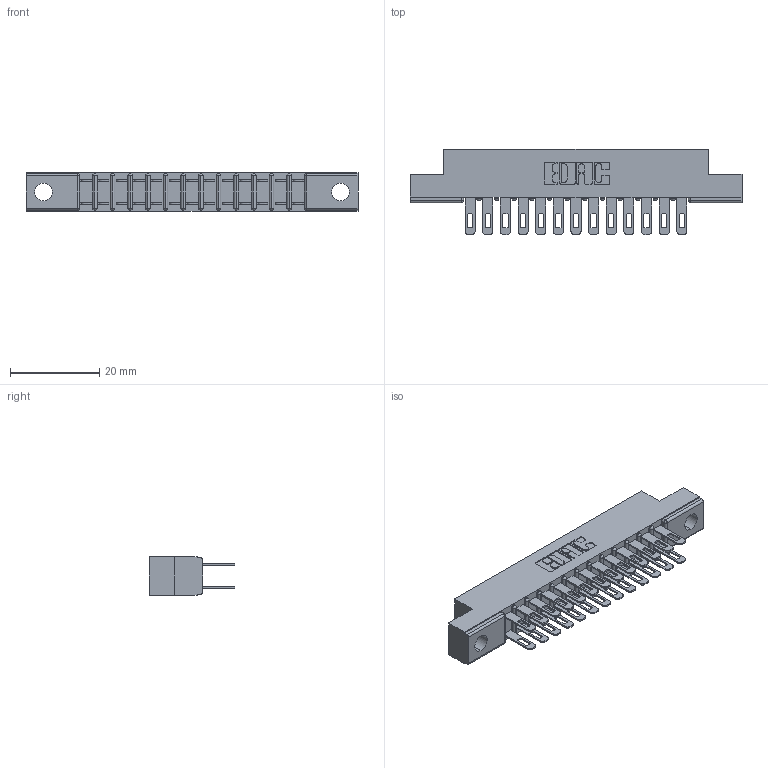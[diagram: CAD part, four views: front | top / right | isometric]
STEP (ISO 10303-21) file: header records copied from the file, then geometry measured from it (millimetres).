
FILE_DESCRIPTION (( 'STEP AP203' ), '1' );
FILE_NAME ('307-026-500-204.STEP', '2019-09-05T22:39:11', ( '' ), ( '' ), 'SwSTEP 2.0', 'SolidWorks 2016', '' );
FILE_SCHEMA (( 'CONFIG_CONTROL_DESIGN' ));
Length unit declared in the file: inch
Products named in the file (3): 307 Part_.156 Dia Mounting Holes; 307-026-500-204; 307-290-001_500
Assembly tree (27 placements, depth 2):
  307-026-500-204
    307 Part_.156 Dia Mounting Holes
    307-290-001_500  x26
Bounding box: 74.52 x 19.18 x 8.71 mm (x, y, z)
Volume: 4844.2 mm3; surface area: 8388.4 mm2
Topology: 27 solids, 27 shells, 1342 faces, 3739 edges, 2418 vertices
Faces by surface type: plane 864, cylinder 450, sphere 28
Entity records: 15528 total; most frequent: CARTESIAN_POINT 2551, ORIENTED_EDGE 2522, DIRECTION 2505, EDGE_CURVE 1261, LINE 961, VECTOR 961, VERTEX_POINT 818, AXIS2_PLACEMENT_3D 772
